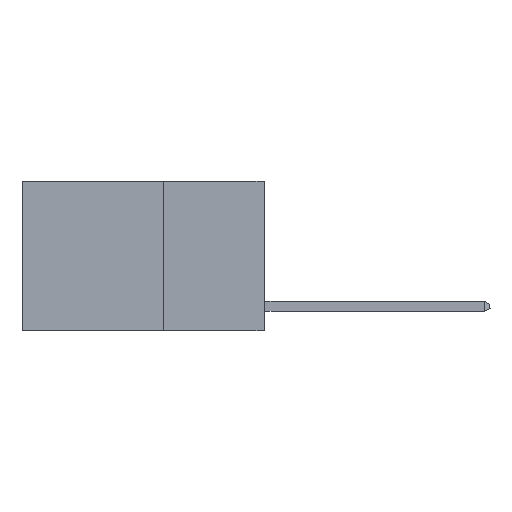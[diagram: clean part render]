
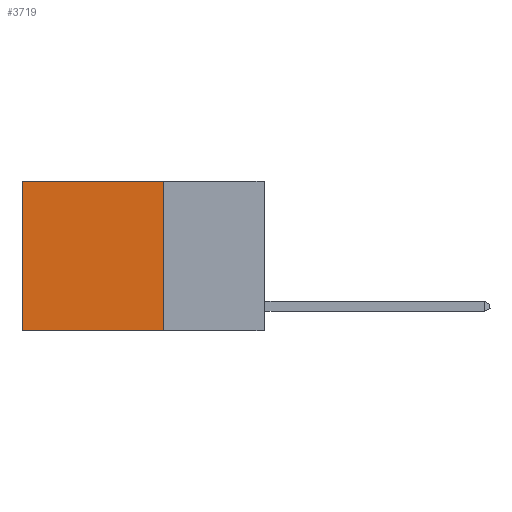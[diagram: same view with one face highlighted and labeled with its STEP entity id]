
A CAD part, left-side view. The second image highlights one B-rep face of the part: STEP entity #3719.
In plain terms, the highlighted planar face has unit normal (-1, 0, 0).
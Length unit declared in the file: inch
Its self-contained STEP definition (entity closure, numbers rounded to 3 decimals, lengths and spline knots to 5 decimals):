
#317 = EDGE_CURVE ( 'NONE', #24738, #5011, #26772, .T. ) ;
#1383 = VERTEX_POINT ( 'NONE', #16485 ) ;
#1454 = ORIENTED_EDGE ( 'NONE', *, *, #22563, .F. ) ;
#1648 = LINE ( 'NONE', #4061, #22560 ) ;
#2352 = CARTESIAN_POINT ( 'NONE',  ( 0.2625, 0.25, 0. ) ) ;
#2360 = DIRECTION ( 'NONE',  ( 0., 0., -1. ) ) ;
#3266 = CARTESIAN_POINT ( 'NONE',  ( 0.2625, 0.25, -0.37 ) ) ;
#3719 = ADVANCED_FACE ( 'NONE', ( #23405 ), #8624, .F. ) ;
#4061 = CARTESIAN_POINT ( 'NONE',  ( 0.2625, 0.25, 0. ) ) ;
#5011 = VERTEX_POINT ( 'NONE', #18990 ) ;
#5382 = DIRECTION ( 'NONE',  ( 0., 1., 0. ) ) ;
#6320 = ORIENTED_EDGE ( 'NONE', *, *, #317, .T. ) ;
#6390 = CARTESIAN_POINT ( 'NONE',  ( 0.2625, 0.25, 0. ) ) ;
#8308 = DIRECTION ( 'NONE',  ( 0., 0., -1. ) ) ;
#8520 = ORIENTED_EDGE ( 'NONE', *, *, #25397, .T. ) ;
#8624 = PLANE ( 'NONE',  #21427 ) ;
#9760 = VECTOR ( 'NONE', #19163, 39.37008 ) ;
#9877 = CARTESIAN_POINT ( 'NONE',  ( 0.2625, 0.25, -0.37 ) ) ;
#11039 = EDGE_LOOP ( 'NONE', ( #8520, #1454, #19914, #6320 ) ) ;
#14933 = DIRECTION ( 'NONE',  ( 1., 0., 0. ) ) ;
#15912 = EDGE_CURVE ( 'NONE', #24738, #26377, #1648, .T. ) ;
#16437 = VECTOR ( 'NONE', #5382, 39.37008 ) ;
#16485 = CARTESIAN_POINT ( 'NONE',  ( 0.2625, 0.6, -0.37 ) ) ;
#16700 = DIRECTION ( 'NONE',  ( 0., 1., 0. ) ) ;
#17070 = CARTESIAN_POINT ( 'NONE',  ( 0.2625, 0.6, 0. ) ) ;
#18990 = CARTESIAN_POINT ( 'NONE',  ( 0.2625, 0.6, 0. ) ) ;
#19163 = DIRECTION ( 'NONE',  ( 0., 0., -1. ) ) ;
#19914 = ORIENTED_EDGE ( 'NONE', *, *, #15912, .F. ) ;
#21101 = CARTESIAN_POINT ( 'NONE',  ( 0.2625, 0.25, 0. ) ) ;
#21236 = VECTOR ( 'NONE', #16700, 39.37008 ) ;
#21427 = AXIS2_PLACEMENT_3D ( 'NONE', #21101, #14933, #2360 ) ;
#22560 = VECTOR ( 'NONE', #8308, 39.37008 ) ;
#22563 = EDGE_CURVE ( 'NONE', #26377, #1383, #26851, .T. ) ;
#23405 = FACE_OUTER_BOUND ( 'NONE', #11039, .T. ) ;
#24738 = VERTEX_POINT ( 'NONE', #2352 ) ;
#25397 = EDGE_CURVE ( 'NONE', #5011, #1383, #26386, .T. ) ;
#26377 = VERTEX_POINT ( 'NONE', #9877 ) ;
#26386 = LINE ( 'NONE', #17070, #9760 ) ;
#26772 = LINE ( 'NONE', #6390, #21236 ) ;
#26851 = LINE ( 'NONE', #3266, #16437 ) ;
